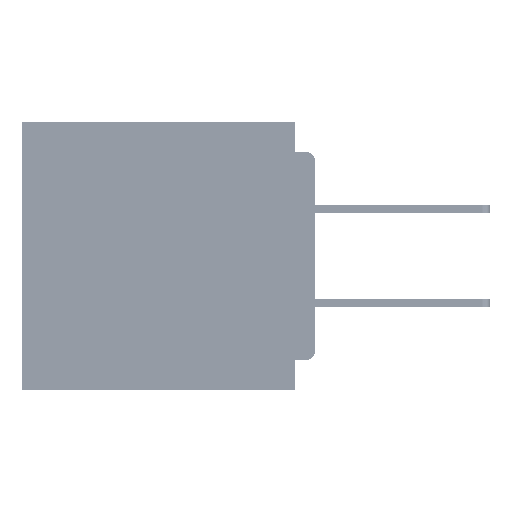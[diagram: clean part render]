
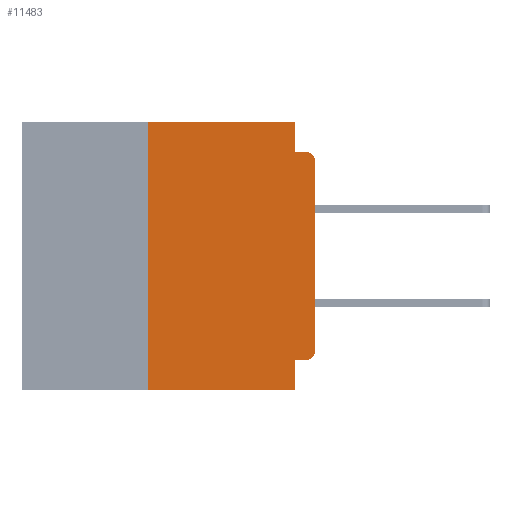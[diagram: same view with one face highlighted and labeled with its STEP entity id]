
A CAD part, left-side view. The second image highlights one B-rep face of the part: STEP entity #11483.
In plain terms, the highlighted planar face has unit normal (-1, 0, 0).
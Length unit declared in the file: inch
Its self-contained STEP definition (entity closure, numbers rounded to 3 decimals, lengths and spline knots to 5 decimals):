
#32 = LINE ( 'NONE', #57776, #26774 ) ;
#96 = VECTOR ( 'NONE', #59011, 39.37008 ) ;
#1062 = AXIS2_PLACEMENT_3D ( 'NONE', #56400, #24596, #61966 ) ;
#1918 = CARTESIAN_POINT ( 'NONE',  ( 0., 0.031, -0.045 ) ) ;
#3605 = CARTESIAN_POINT ( 'NONE',  ( 0., 0.015, -0.355 ) ) ;
#4017 = CIRCLE ( 'NONE', #58006, 0.015 ) ;
#5217 = DIRECTION ( 'NONE',  ( 0., 1., 0. ) ) ;
#9069 = ORIENTED_EDGE ( 'NONE', *, *, #20237, .F. ) ;
#11483 = ADVANCED_FACE ( 'NONE', ( #27107 ), #13853, .F. ) ;
#12422 = AXIS2_PLACEMENT_3D ( 'NONE', #19514, #56934, #24894 ) ;
#13829 = EDGE_CURVE ( 'NONE', #45695, #63231, #31851, .T. ) ;
#13853 = PLANE ( 'NONE',  #1062 ) ;
#14746 = CARTESIAN_POINT ( 'NONE',  ( 0., 0.25, 0. ) ) ;
#15842 = CIRCLE ( 'NONE', #12422, 0.015 ) ;
#15980 = EDGE_CURVE ( 'NONE', #68488, #32665, #42387, .T. ) ;
#17367 = DIRECTION ( 'NONE',  ( -1., 0., 0. ) ) ;
#17893 = CARTESIAN_POINT ( 'NONE',  ( 0., 0.031, -0.355 ) ) ;
#18914 = EDGE_CURVE ( 'NONE', #69215, #32930, #32, .T. ) ;
#19178 = DIRECTION ( 'NONE',  ( 0., -1., 0. ) ) ;
#19468 = LINE ( 'NONE', #45618, #47835 ) ;
#19514 = CARTESIAN_POINT ( 'NONE',  ( 0., 0.015, -0.34 ) ) ;
#20237 = EDGE_CURVE ( 'NONE', #36909, #68488, #55044, .T. ) ;
#20425 = EDGE_CURVE ( 'NONE', #34659, #40729, #4017, .T. ) ;
#24207 = ORIENTED_EDGE ( 'NONE', *, *, #15980, .F. ) ;
#24596 = DIRECTION ( 'NONE',  ( 1., 0., 0. ) ) ;
#24894 = DIRECTION ( 'NONE',  ( 0., 0., -1. ) ) ;
#26774 = VECTOR ( 'NONE', #36462, 39.37008 ) ;
#26982 = CARTESIAN_POINT ( 'NONE',  ( 0., 0.25, -0.4 ) ) ;
#27107 = FACE_OUTER_BOUND ( 'NONE', #61626, .T. ) ;
#28690 = VECTOR ( 'NONE', #49443, 39.37008 ) ;
#29677 = EDGE_CURVE ( 'NONE', #45695, #32665, #61365, .T. ) ;
#30347 = LINE ( 'NONE', #33310, #28690 ) ;
#31051 = CARTESIAN_POINT ( 'NONE',  ( 0., 0.015, -0.045 ) ) ;
#31851 = LINE ( 'NONE', #26982, #96 ) ;
#32665 = VERTEX_POINT ( 'NONE', #53364 ) ;
#32930 = VERTEX_POINT ( 'NONE', #1918 ) ;
#33310 = CARTESIAN_POINT ( 'NONE',  ( 0., 0., -0.045 ) ) ;
#33486 = ORIENTED_EDGE ( 'NONE', *, *, #44192, .T. ) ;
#34137 = CARTESIAN_POINT ( 'NONE',  ( 0., 0., -0.06 ) ) ;
#34659 = VERTEX_POINT ( 'NONE', #34137 ) ;
#34884 = VERTEX_POINT ( 'NONE', #35751 ) ;
#35217 = CARTESIAN_POINT ( 'NONE',  ( 0., 0.031, -0.4 ) ) ;
#35388 = ORIENTED_EDGE ( 'NONE', *, *, #13829, .F. ) ;
#35751 = CARTESIAN_POINT ( 'NONE',  ( 0., 0., -0.34 ) ) ;
#36462 = DIRECTION ( 'NONE',  ( 0., 0., -1. ) ) ;
#36841 = EDGE_CURVE ( 'NONE', #63231, #69215, #19468, .T. ) ;
#36909 = VERTEX_POINT ( 'NONE', #3605 ) ;
#37209 = CARTESIAN_POINT ( 'NONE',  ( 0., 0., -0.355 ) ) ;
#38233 = ORIENTED_EDGE ( 'NONE', *, *, #18914, .F. ) ;
#40729 = VERTEX_POINT ( 'NONE', #31051 ) ;
#40788 = VECTOR ( 'NONE', #5217, 39.37008 ) ;
#42387 = LINE ( 'NONE', #35217, #56671 ) ;
#44192 = EDGE_CURVE ( 'NONE', #34884, #34659, #48791, .T. ) ;
#44407 = EDGE_CURVE ( 'NONE', #32930, #40729, #30347, .T. ) ;
#45433 = VECTOR ( 'NONE', #19178, 39.37008 ) ;
#45618 = CARTESIAN_POINT ( 'NONE',  ( 0., 0.437, 0. ) ) ;
#45695 = VERTEX_POINT ( 'NONE', #50813 ) ;
#45843 = DIRECTION ( 'NONE',  ( 0., -1., 0. ) ) ;
#47773 = ORIENTED_EDGE ( 'NONE', *, *, #20425, .T. ) ;
#47835 = VECTOR ( 'NONE', #45843, 39.37008 ) ;
#48791 = LINE ( 'NONE', #52758, #59694 ) ;
#49334 = CARTESIAN_POINT ( 'NONE',  ( 0., 0.015, -0.06 ) ) ;
#49443 = DIRECTION ( 'NONE',  ( 0., -1., 0. ) ) ;
#50112 = ORIENTED_EDGE ( 'NONE', *, *, #56329, .T. ) ;
#50813 = CARTESIAN_POINT ( 'NONE',  ( 0., 0.25, -0.4 ) ) ;
#52758 = CARTESIAN_POINT ( 'NONE',  ( 0., 0., 0. ) ) ;
#53364 = CARTESIAN_POINT ( 'NONE',  ( 0., 0.031, -0.4 ) ) ;
#54761 = DIRECTION ( 'NONE',  ( 0., 0., -1. ) ) ;
#55044 = LINE ( 'NONE', #37209, #40788 ) ;
#55891 = CARTESIAN_POINT ( 'NONE',  ( 0., 0.031, 0. ) ) ;
#56329 = EDGE_CURVE ( 'NONE', #36909, #34884, #15842, .T. ) ;
#56400 = CARTESIAN_POINT ( 'NONE',  ( 0., 0.437, 0. ) ) ;
#56588 = CARTESIAN_POINT ( 'NONE',  ( 0., 0.437, -0.4 ) ) ;
#56671 = VECTOR ( 'NONE', #67242, 39.37008 ) ;
#56934 = DIRECTION ( 'NONE',  ( -1., 0., 0. ) ) ;
#57776 = CARTESIAN_POINT ( 'NONE',  ( 0., 0.031, 0. ) ) ;
#58006 = AXIS2_PLACEMENT_3D ( 'NONE', #49334, #17367, #54761 ) ;
#58585 = ORIENTED_EDGE ( 'NONE', *, *, #29677, .T. ) ;
#59011 = DIRECTION ( 'NONE',  ( 0., 0., 1. ) ) ;
#59694 = VECTOR ( 'NONE', #68868, 39.37008 ) ;
#61365 = LINE ( 'NONE', #56588, #45433 ) ;
#61626 = EDGE_LOOP ( 'NONE', ( #33486, #47773, #65080, #38233, #66181, #35388, #58585, #24207, #9069, #50112 ) ) ;
#61966 = DIRECTION ( 'NONE',  ( 0., 0., -1. ) ) ;
#63231 = VERTEX_POINT ( 'NONE', #14746 ) ;
#65080 = ORIENTED_EDGE ( 'NONE', *, *, #44407, .F. ) ;
#66181 = ORIENTED_EDGE ( 'NONE', *, *, #36841, .F. ) ;
#67242 = DIRECTION ( 'NONE',  ( 0., 0., -1. ) ) ;
#68488 = VERTEX_POINT ( 'NONE', #17893 ) ;
#68868 = DIRECTION ( 'NONE',  ( 0., 0., 1. ) ) ;
#69215 = VERTEX_POINT ( 'NONE', #55891 ) ;
